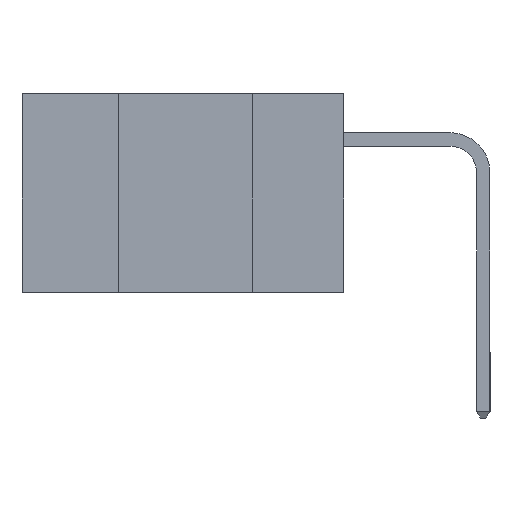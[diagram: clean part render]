
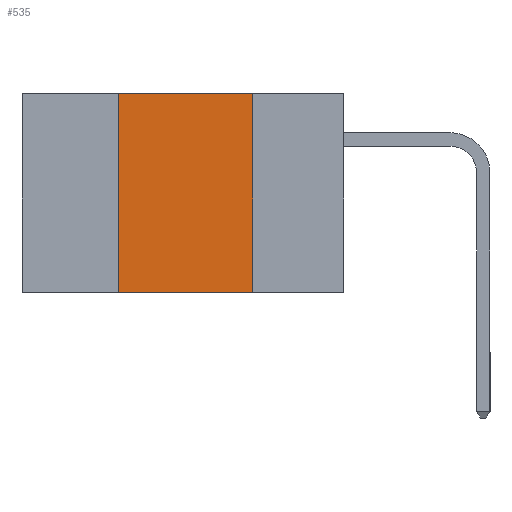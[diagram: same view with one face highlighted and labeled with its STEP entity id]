
A CAD part, left-side view. The second image highlights one B-rep face of the part: STEP entity #535.
In plain terms, the highlighted planar face has unit normal (-1, 0, 0).
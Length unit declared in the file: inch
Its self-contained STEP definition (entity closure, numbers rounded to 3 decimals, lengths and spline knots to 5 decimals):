
#485 = CARTESIAN_POINT ( 'NONE',  ( 0., 0.17, -0.37 ) ) ;
#535 = ADVANCED_FACE ( 'NONE', ( #21835 ), #6435, .F. ) ;
#2569 = VECTOR ( 'NONE', #21119, 39.37008 ) ;
#2616 = DIRECTION ( 'NONE',  ( 0., 0., 1. ) ) ;
#2975 = DIRECTION ( 'NONE',  ( 1., 0., 0. ) ) ;
#3402 = ORIENTED_EDGE ( 'NONE', *, *, #4693, .F. ) ;
#3713 = DIRECTION ( 'NONE',  ( 0., -1., 0. ) ) ;
#4278 = LINE ( 'NONE', #21850, #21346 ) ;
#4441 = DIRECTION ( 'NONE',  ( 0., -1., 0. ) ) ;
#4646 = DIRECTION ( 'NONE',  ( 0., 0., -1. ) ) ;
#4693 = EDGE_CURVE ( 'NONE', #17938, #20305, #4278, .T. ) ;
#6435 = PLANE ( 'NONE',  #15274 ) ;
#7986 = LINE ( 'NONE', #23270, #2569 ) ;
#8640 = EDGE_LOOP ( 'NONE', ( #10304, #14862, #3402, #22808 ) ) ;
#8694 = CARTESIAN_POINT ( 'NONE',  ( 0., 0.42, -0.37 ) ) ;
#9136 = EDGE_CURVE ( 'NONE', #17938, #24738, #20095, .T. ) ;
#10304 = ORIENTED_EDGE ( 'NONE', *, *, #22956, .F. ) ;
#11489 = CARTESIAN_POINT ( 'NONE',  ( 0., 0.6, 0. ) ) ;
#12589 = CARTESIAN_POINT ( 'NONE',  ( 0., 0.6, -0.37 ) ) ;
#14011 = VECTOR ( 'NONE', #3713, 39.37008 ) ;
#14862 = ORIENTED_EDGE ( 'NONE', *, *, #24487, .F. ) ;
#15274 = AXIS2_PLACEMENT_3D ( 'NONE', #20421, #2975, #4646 ) ;
#17465 = VERTEX_POINT ( 'NONE', #21598 ) ;
#17938 = VERTEX_POINT ( 'NONE', #8694 ) ;
#20095 = LINE ( 'NONE', #12589, #23480 ) ;
#20305 = VERTEX_POINT ( 'NONE', #20851 ) ;
#20421 = CARTESIAN_POINT ( 'NONE',  ( 0., 0.6, 0. ) ) ;
#20851 = CARTESIAN_POINT ( 'NONE',  ( 0., 0.42, 0. ) ) ;
#21119 = DIRECTION ( 'NONE',  ( 0., 0., -1. ) ) ;
#21346 = VECTOR ( 'NONE', #2616, 39.37008 ) ;
#21598 = CARTESIAN_POINT ( 'NONE',  ( 0., 0.17, 0. ) ) ;
#21835 = FACE_OUTER_BOUND ( 'NONE', #8640, .T. ) ;
#21850 = CARTESIAN_POINT ( 'NONE',  ( 0., 0.42, -0.37 ) ) ;
#22808 = ORIENTED_EDGE ( 'NONE', *, *, #9136, .T. ) ;
#22956 = EDGE_CURVE ( 'NONE', #17465, #24738, #7986, .T. ) ;
#23070 = LINE ( 'NONE', #11489, #14011 ) ;
#23270 = CARTESIAN_POINT ( 'NONE',  ( 0., 0.17, -0.37 ) ) ;
#23480 = VECTOR ( 'NONE', #4441, 39.37008 ) ;
#24487 = EDGE_CURVE ( 'NONE', #20305, #17465, #23070, .T. ) ;
#24738 = VERTEX_POINT ( 'NONE', #485 ) ;
